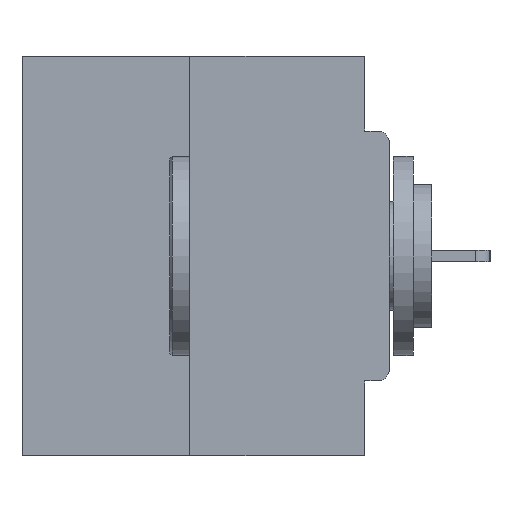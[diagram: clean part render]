
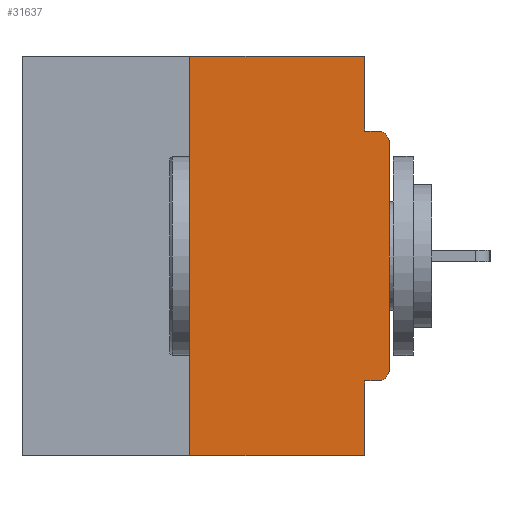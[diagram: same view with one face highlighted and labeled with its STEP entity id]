
A CAD part, left-side view. The second image highlights one B-rep face of the part: STEP entity #31637.
In plain terms, the highlighted planar face has unit normal (-1, 0, 0).
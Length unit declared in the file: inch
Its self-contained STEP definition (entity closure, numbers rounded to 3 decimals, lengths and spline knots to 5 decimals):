
#368 = VERTEX_POINT ( 'NONE', #16339 ) ;
#539 = CARTESIAN_POINT ( 'NONE',  ( 0., 0., -0.3915 ) ) ;
#1211 = VECTOR ( 'NONE', #29121, 39.37008 ) ;
#1700 = CARTESIAN_POINT ( 'NONE',  ( 0., 0.015, -0.0935 ) ) ;
#2213 = DIRECTION ( 'NONE',  ( -1., 0., 0. ) ) ;
#4070 = VECTOR ( 'NONE', #31070, 39.37008 ) ;
#5494 = LINE ( 'NONE', #17608, #17811 ) ;
#5539 = EDGE_CURVE ( 'NONE', #19617, #11899, #25604, .T. ) ;
#5733 = VECTOR ( 'NONE', #19536, 39.37008 ) ;
#6227 = CARTESIAN_POINT ( 'NONE',  ( 0., 0.015, -0.4065 ) ) ;
#6265 = CIRCLE ( 'NONE', #14303, 0.015 ) ;
#6406 = CARTESIAN_POINT ( 'NONE',  ( 0., 0.031, 0. ) ) ;
#6678 = CARTESIAN_POINT ( 'NONE',  ( 0., 0.031, -0.0935 ) ) ;
#6854 = CARTESIAN_POINT ( 'NONE',  ( 0., 0.031, -0.5 ) ) ;
#8152 = EDGE_CURVE ( 'NONE', #21550, #27956, #17214, .T. ) ;
#8664 = DIRECTION ( 'NONE',  ( 0., 0., -1. ) ) ;
#8862 = EDGE_CURVE ( 'NONE', #29485, #27219, #27652, .T. ) ;
#8966 = EDGE_CURVE ( 'NONE', #31502, #368, #25321, .T. ) ;
#9474 = ORIENTED_EDGE ( 'NONE', *, *, #8966, .T. ) ;
#9616 = CARTESIAN_POINT ( 'NONE',  ( 0., 0., 0. ) ) ;
#9701 = CARTESIAN_POINT ( 'NONE',  ( 0., 0.25, 0. ) ) ;
#9755 = CARTESIAN_POINT ( 'NONE',  ( 0., 0.031, 0. ) ) ;
#10056 = CARTESIAN_POINT ( 'NONE',  ( 0., 0.015, -0.1085 ) ) ;
#10540 = CARTESIAN_POINT ( 'NONE',  ( 0., 0.46, -0.5 ) ) ;
#11096 = ORIENTED_EDGE ( 'NONE', *, *, #8862, .F. ) ;
#11124 = VERTEX_POINT ( 'NONE', #6227 ) ;
#11390 = VECTOR ( 'NONE', #29420, 39.37008 ) ;
#11899 = VERTEX_POINT ( 'NONE', #1700 ) ;
#12044 = CARTESIAN_POINT ( 'NONE',  ( 0., 0.46, 0. ) ) ;
#12533 = DIRECTION ( 'NONE',  ( 0., 0., -1. ) ) ;
#14063 = EDGE_CURVE ( 'NONE', #11124, #31502, #6265, .T. ) ;
#14279 = CARTESIAN_POINT ( 'NONE',  ( 0., 0.031, -0.5 ) ) ;
#14303 = AXIS2_PLACEMENT_3D ( 'NONE', #17111, #2213, #19545 ) ;
#14753 = EDGE_CURVE ( 'NONE', #11124, #29485, #5494, .T. ) ;
#16339 = CARTESIAN_POINT ( 'NONE',  ( 0., 0., -0.1085 ) ) ;
#16479 = ORIENTED_EDGE ( 'NONE', *, *, #30640, .F. ) ;
#16832 = LINE ( 'NONE', #12044, #23451 ) ;
#17111 = CARTESIAN_POINT ( 'NONE',  ( 0., 0.015, -0.3915 ) ) ;
#17214 = LINE ( 'NONE', #18611, #4070 ) ;
#17596 = ORIENTED_EDGE ( 'NONE', *, *, #17643, .T. ) ;
#17608 = CARTESIAN_POINT ( 'NONE',  ( 0., 0., -0.4065 ) ) ;
#17643 = EDGE_CURVE ( 'NONE', #368, #11899, #22271, .T. ) ;
#17811 = VECTOR ( 'NONE', #22626, 39.37008 ) ;
#18611 = CARTESIAN_POINT ( 'NONE',  ( 0., 0.25, 0. ) ) ;
#19409 = EDGE_LOOP ( 'NONE', ( #16479, #19517, #28540, #11096, #30806, #27694, #9474, #17596, #30401, #31158 ) ) ;
#19517 = ORIENTED_EDGE ( 'NONE', *, *, #8152, .F. ) ;
#19536 = DIRECTION ( 'NONE',  ( 0., 0., -1. ) ) ;
#19545 = DIRECTION ( 'NONE',  ( 0., 0., -1. ) ) ;
#19617 = VERTEX_POINT ( 'NONE', #6678 ) ;
#20978 = CARTESIAN_POINT ( 'NONE',  ( 0., 0.46, 0. ) ) ;
#21550 = VERTEX_POINT ( 'NONE', #23261 ) ;
#21741 = CARTESIAN_POINT ( 'NONE',  ( 0., 0.031, -0.4065 ) ) ;
#22271 = CIRCLE ( 'NONE', #30342, 0.015 ) ;
#22618 = EDGE_CURVE ( 'NONE', #27730, #19617, #26215, .T. ) ;
#22626 = DIRECTION ( 'NONE',  ( 0., 1., 0. ) ) ;
#23261 = CARTESIAN_POINT ( 'NONE',  ( 0., 0.25, -0.5 ) ) ;
#23451 = VECTOR ( 'NONE', #26891, 39.37008 ) ;
#23496 = DIRECTION ( 'NONE',  ( 1., 0., 0. ) ) ;
#23544 = CARTESIAN_POINT ( 'NONE',  ( 0., 0., -0.0935 ) ) ;
#24821 = VECTOR ( 'NONE', #25189, 39.37008 ) ;
#25189 = DIRECTION ( 'NONE',  ( 0., -1., 0. ) ) ;
#25300 = FACE_OUTER_BOUND ( 'NONE', #19409, .T. ) ;
#25321 = LINE ( 'NONE', #9616, #11390 ) ;
#25354 = DIRECTION ( 'NONE',  ( 0., -1., 0. ) ) ;
#25485 = VECTOR ( 'NONE', #25354, 39.37008 ) ;
#25604 = LINE ( 'NONE', #23544, #24821 ) ;
#25874 = PLANE ( 'NONE',  #28165 ) ;
#26215 = LINE ( 'NONE', #9755, #5733 ) ;
#26891 = DIRECTION ( 'NONE',  ( 0., -1., 0. ) ) ;
#27219 = VERTEX_POINT ( 'NONE', #6854 ) ;
#27364 = DIRECTION ( 'NONE',  ( -1., 0., 0. ) ) ;
#27652 = LINE ( 'NONE', #14279, #1211 ) ;
#27694 = ORIENTED_EDGE ( 'NONE', *, *, #14063, .T. ) ;
#27730 = VERTEX_POINT ( 'NONE', #6406 ) ;
#27956 = VERTEX_POINT ( 'NONE', #9701 ) ;
#28165 = AXIS2_PLACEMENT_3D ( 'NONE', #20978, #23496, #8664 ) ;
#28540 = ORIENTED_EDGE ( 'NONE', *, *, #28740, .T. ) ;
#28740 = EDGE_CURVE ( 'NONE', #21550, #27219, #31247, .T. ) ;
#29121 = DIRECTION ( 'NONE',  ( 0., 0., -1. ) ) ;
#29420 = DIRECTION ( 'NONE',  ( 0., 0., 1. ) ) ;
#29485 = VERTEX_POINT ( 'NONE', #21741 ) ;
#30342 = AXIS2_PLACEMENT_3D ( 'NONE', #10056, #27364, #12533 ) ;
#30401 = ORIENTED_EDGE ( 'NONE', *, *, #5539, .F. ) ;
#30640 = EDGE_CURVE ( 'NONE', #27956, #27730, #16832, .T. ) ;
#30806 = ORIENTED_EDGE ( 'NONE', *, *, #14753, .F. ) ;
#31070 = DIRECTION ( 'NONE',  ( 0., 0., 1. ) ) ;
#31158 = ORIENTED_EDGE ( 'NONE', *, *, #22618, .F. ) ;
#31247 = LINE ( 'NONE', #10540, #25485 ) ;
#31502 = VERTEX_POINT ( 'NONE', #539 ) ;
#31637 = ADVANCED_FACE ( 'NONE', ( #25300 ), #25874, .F. ) ;
